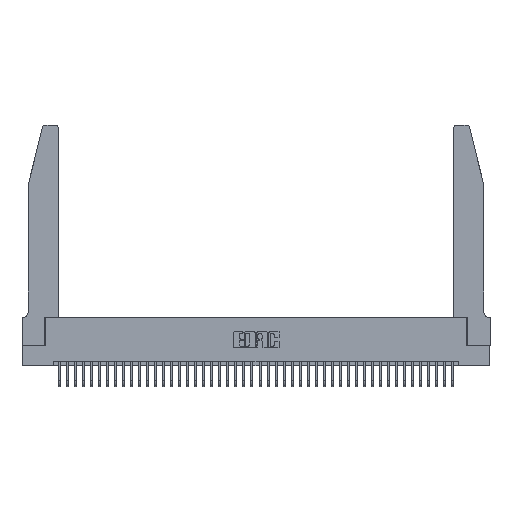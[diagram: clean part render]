
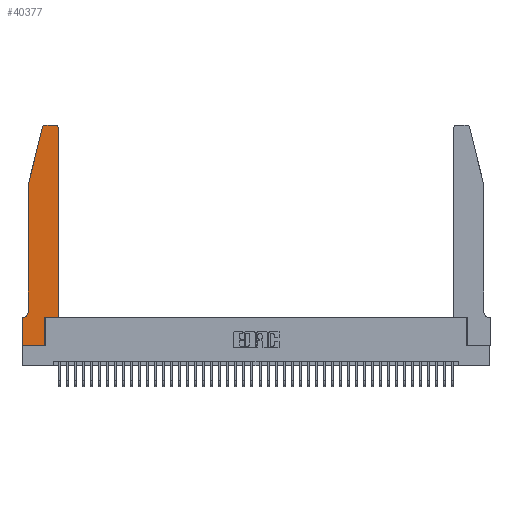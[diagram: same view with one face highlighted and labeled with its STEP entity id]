
A CAD part, top view. The second image highlights one B-rep face of the part: STEP entity #40377.
In plain terms, the highlighted planar face has unit normal (0, 0, 1).
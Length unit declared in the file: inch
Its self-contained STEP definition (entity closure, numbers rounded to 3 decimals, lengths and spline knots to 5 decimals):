
#54 = AXIS2_PLACEMENT_3D ( 'NONE', #4396, #36370, #17230 ) ;
#449 = EDGE_CURVE ( 'NONE', #20316, #38186, #15812, .T. ) ;
#1350 = CIRCLE ( 'NONE', #36254, 0.07 ) ;
#1906 = DIRECTION ( 'NONE',  ( -0.239, -0.971, 0. ) ) ;
#2198 = ORIENTED_EDGE ( 'NONE', *, *, #449, .T. ) ;
#2330 = VERTEX_POINT ( 'NONE', #22564 ) ;
#2380 = FACE_OUTER_BOUND ( 'NONE', #10137, .T. ) ;
#2535 = VERTEX_POINT ( 'NONE', #4315 ) ;
#2577 = CARTESIAN_POINT ( 'NONE',  ( 0.0055, 0.42, 0.37 ) ) ;
#2743 = DIRECTION ( 'NONE',  ( 0., 1., 0. ) ) ;
#3048 = CARTESIAN_POINT ( 'NONE',  ( 0.2865, 0.35, 0.37 ) ) ;
#3606 = LINE ( 'NONE', #18366, #36585 ) ;
#4315 = CARTESIAN_POINT ( 'NONE',  ( 0.4205, 2.75, 0.37 ) ) ;
#4396 = CARTESIAN_POINT ( 'NONE',  ( 0., 0.35, 0.37 ) ) ;
#4958 = CARTESIAN_POINT ( 'NONE',  ( 0.284, 2.75, 0.37 ) ) ;
#4990 = CARTESIAN_POINT ( 'NONE',  ( 0.4505, 0.35, 0.37 ) ) ;
#5085 = CARTESIAN_POINT ( 'NONE',  ( 0.25487, 2.72718, 0.37 ) ) ;
#5618 = VECTOR ( 'NONE', #36693, 39.37008 ) ;
#5828 = DIRECTION ( 'NONE',  ( -1., 0., 0. ) ) ;
#6111 = DIRECTION ( 'NONE',  ( 0., 1., 0. ) ) ;
#7316 = VECTOR ( 'NONE', #34809, 39.37008 ) ;
#7812 = CIRCLE ( 'NONE', #27362, 0.03 ) ;
#9094 = EDGE_CURVE ( 'NONE', #2330, #25557, #22641, .T. ) ;
#10137 = EDGE_LOOP ( 'NONE', ( #35520, #38842, #24563, #34049, #38284, #2198, #26259, #28793, #24193, #35144, #13064, #41253 ) ) ;
#11082 = EDGE_CURVE ( 'NONE', #26804, #16202, #32082, .T. ) ;
#11394 = VECTOR ( 'NONE', #32720, 39.37008 ) ;
#11661 = VERTEX_POINT ( 'NONE', #5085 ) ;
#11694 = CARTESIAN_POINT ( 'NONE',  ( 0., 0., 0.37 ) ) ;
#13064 = ORIENTED_EDGE ( 'NONE', *, *, #29002, .T. ) ;
#13950 = VECTOR ( 'NONE', #17694, 39.37008 ) ;
#14725 = CARTESIAN_POINT ( 'NONE',  ( 0.4205, 2.72, 0.37 ) ) ;
#14874 = EDGE_CURVE ( 'NONE', #16202, #16355, #29294, .T. ) ;
#15575 = CARTESIAN_POINT ( 'NONE',  ( 0.4505, 0.35, 0.37 ) ) ;
#15812 = LINE ( 'NONE', #37994, #7316 ) ;
#16048 = VECTOR ( 'NONE', #37229, 39.37008 ) ;
#16130 = VECTOR ( 'NONE', #6111, 39.37008 ) ;
#16202 = VERTEX_POINT ( 'NONE', #31034 ) ;
#16355 = VERTEX_POINT ( 'NONE', #3048 ) ;
#17230 = DIRECTION ( 'NONE',  ( 1., 0., 0. ) ) ;
#17234 = CARTESIAN_POINT ( 'NONE',  ( 0.4505, 2.72, 0.37 ) ) ;
#17694 = DIRECTION ( 'NONE',  ( 1., 0., 0. ) ) ;
#17854 = CARTESIAN_POINT ( 'NONE',  ( 0.0755, 2., 0.37 ) ) ;
#17938 = DIRECTION ( 'NONE',  ( 1., 0., 0. ) ) ;
#18366 = CARTESIAN_POINT ( 'NONE',  ( 0.2605, 2.75, 0.37 ) ) ;
#19151 = CARTESIAN_POINT ( 'NONE',  ( 0.284, 2.72, 0.37 ) ) ;
#19776 = VECTOR ( 'NONE', #2743, 39.37008 ) ;
#19878 = LINE ( 'NONE', #39093, #11394 ) ;
#20316 = VERTEX_POINT ( 'NONE', #34887 ) ;
#21371 = CIRCLE ( 'NONE', #36882, 0.03 ) ;
#22405 = DIRECTION ( 'NONE',  ( 1., 0., 0. ) ) ;
#22564 = CARTESIAN_POINT ( 'NONE',  ( 0.0755, 2., 0.37 ) ) ;
#22641 = LINE ( 'NONE', #33490, #5618 ) ;
#22998 = EDGE_CURVE ( 'NONE', #38186, #26804, #19878, .T. ) ;
#23589 = PLANE ( 'NONE',  #54 ) ;
#24193 = ORIENTED_EDGE ( 'NONE', *, *, #14874, .T. ) ;
#24563 = ORIENTED_EDGE ( 'NONE', *, *, #34468, .T. ) ;
#24992 = DIRECTION ( 'NONE',  ( 0., 0., -1. ) ) ;
#25557 = VERTEX_POINT ( 'NONE', #40708 ) ;
#26094 = EDGE_CURVE ( 'NONE', #2535, #33333, #3606, .T. ) ;
#26259 = ORIENTED_EDGE ( 'NONE', *, *, #22998, .T. ) ;
#26804 = VERTEX_POINT ( 'NONE', #27080 ) ;
#27080 = CARTESIAN_POINT ( 'NONE',  ( 0., 0., 0.37 ) ) ;
#27362 = AXIS2_PLACEMENT_3D ( 'NONE', #19151, #40261, #22405 ) ;
#28043 = DIRECTION ( 'NONE',  ( -1., 0., 0. ) ) ;
#28768 = VERTEX_POINT ( 'NONE', #4990 ) ;
#28793 = ORIENTED_EDGE ( 'NONE', *, *, #11082, .T. ) ;
#28969 = LINE ( 'NONE', #36833, #13950 ) ;
#29002 = EDGE_CURVE ( 'NONE', #28768, #30872, #33147, .T. ) ;
#29294 = LINE ( 'NONE', #40980, #19776 ) ;
#29505 = VECTOR ( 'NONE', #1906, 39.37008 ) ;
#30872 = VERTEX_POINT ( 'NONE', #17234 ) ;
#31034 = CARTESIAN_POINT ( 'NONE',  ( 0.2865, 0., 0.37 ) ) ;
#32082 = LINE ( 'NONE', #11694, #16048 ) ;
#32720 = DIRECTION ( 'NONE',  ( 0., -1., 0. ) ) ;
#33147 = LINE ( 'NONE', #15575, #16130 ) ;
#33333 = VERTEX_POINT ( 'NONE', #4958 ) ;
#33365 = EDGE_CURVE ( 'NONE', #30872, #2535, #21371, .T. ) ;
#33490 = CARTESIAN_POINT ( 'NONE',  ( 0.0755, 2., 0.37 ) ) ;
#34049 = ORIENTED_EDGE ( 'NONE', *, *, #9094, .T. ) ;
#34468 = EDGE_CURVE ( 'NONE', #11661, #2330, #38938, .T. ) ;
#34809 = DIRECTION ( 'NONE',  ( -1., 0., 0. ) ) ;
#34887 = CARTESIAN_POINT ( 'NONE',  ( 0.0055, 0.35, 0.37 ) ) ;
#35144 = ORIENTED_EDGE ( 'NONE', *, *, #35845, .T. ) ;
#35520 = ORIENTED_EDGE ( 'NONE', *, *, #26094, .T. ) ;
#35845 = EDGE_CURVE ( 'NONE', #16355, #28768, #28969, .T. ) ;
#36254 = AXIS2_PLACEMENT_3D ( 'NONE', #2577, #24992, #5828 ) ;
#36370 = DIRECTION ( 'NONE',  ( 0., 0., 1. ) ) ;
#36585 = VECTOR ( 'NONE', #28043, 39.37008 ) ;
#36693 = DIRECTION ( 'NONE',  ( 0., -1., 0. ) ) ;
#36833 = CARTESIAN_POINT ( 'NONE',  ( 0.4505, 0.35, 0.37 ) ) ;
#36839 = CARTESIAN_POINT ( 'NONE',  ( 0., 0.35, 0.37 ) ) ;
#36882 = AXIS2_PLACEMENT_3D ( 'NONE', #14725, #37058, #17938 ) ;
#37058 = DIRECTION ( 'NONE',  ( 0., 0., 1. ) ) ;
#37229 = DIRECTION ( 'NONE',  ( 1., 0., 0. ) ) ;
#37280 = EDGE_CURVE ( 'NONE', #33333, #11661, #7812, .T. ) ;
#37994 = CARTESIAN_POINT ( 'NONE',  ( 0.0755, 0.35, 0.37 ) ) ;
#38186 = VERTEX_POINT ( 'NONE', #36839 ) ;
#38284 = ORIENTED_EDGE ( 'NONE', *, *, #41089, .T. ) ;
#38842 = ORIENTED_EDGE ( 'NONE', *, *, #37280, .T. ) ;
#38938 = LINE ( 'NONE', #17854, #29505 ) ;
#39093 = CARTESIAN_POINT ( 'NONE',  ( 0., 0., 0.37 ) ) ;
#40261 = DIRECTION ( 'NONE',  ( 0., 0., 1. ) ) ;
#40377 = ADVANCED_FACE ( 'NONE', ( #2380 ), #23589, .T. ) ;
#40708 = CARTESIAN_POINT ( 'NONE',  ( 0.0755, 0.42, 0.37 ) ) ;
#40980 = CARTESIAN_POINT ( 'NONE',  ( 0.2865, 0.35, 0.37 ) ) ;
#41089 = EDGE_CURVE ( 'NONE', #25557, #20316, #1350, .T. ) ;
#41253 = ORIENTED_EDGE ( 'NONE', *, *, #33365, .T. ) ;
